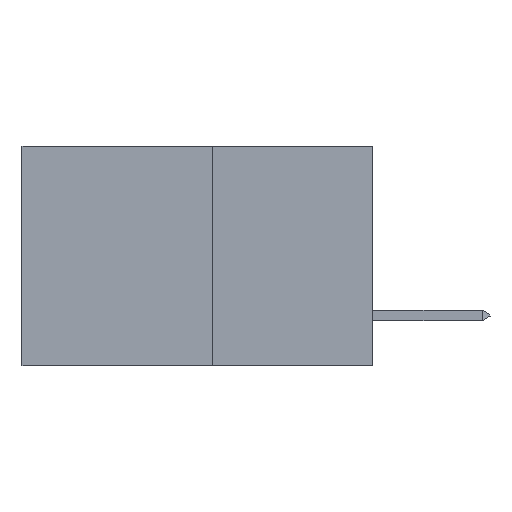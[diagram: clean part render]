
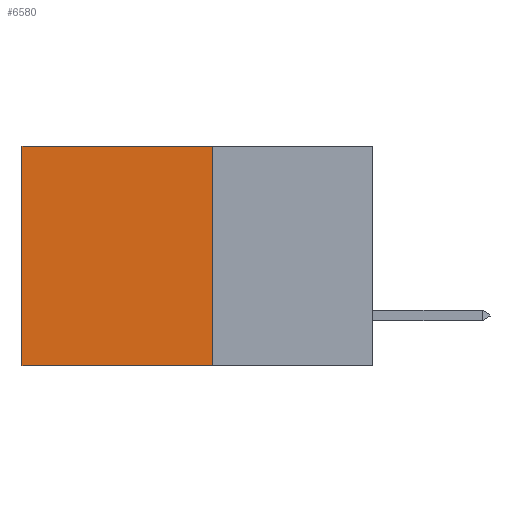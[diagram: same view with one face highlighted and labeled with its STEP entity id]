
A CAD part, left-side view. The second image highlights one B-rep face of the part: STEP entity #6580.
In plain terms, the highlighted planar face has unit normal (-1, 0, 0).
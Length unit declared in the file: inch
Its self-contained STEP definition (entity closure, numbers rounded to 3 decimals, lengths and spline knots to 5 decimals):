
#209 = CARTESIAN_POINT ( 'NONE',  ( 0.277, 0.27, 0. ) ) ;
#249 = VERTEX_POINT ( 'NONE', #7115 ) ;
#510 = CARTESIAN_POINT ( 'NONE',  ( 0.277, 0.59, -0.37 ) ) ;
#636 = DIRECTION ( 'NONE',  ( 0., 0., -1. ) ) ;
#1136 = VECTOR ( 'NONE', #2604, 39.37008 ) ;
#1206 = DIRECTION ( 'NONE',  ( 0., 1., 0. ) ) ;
#1592 = CARTESIAN_POINT ( 'NONE',  ( 0.277, 0.27, -0.37 ) ) ;
#1819 = VERTEX_POINT ( 'NONE', #1592 ) ;
#1961 = LINE ( 'NONE', #8917, #9792 ) ;
#2604 = DIRECTION ( 'NONE',  ( 0., 1., 0. ) ) ;
#2756 = VECTOR ( 'NONE', #636, 39.37008 ) ;
#2848 = CARTESIAN_POINT ( 'NONE',  ( 0.277, 0.27, -0.37 ) ) ;
#3018 = DIRECTION ( 'NONE',  ( 0., 0., -1. ) ) ;
#3955 = CARTESIAN_POINT ( 'NONE',  ( 0.277, 0.27, 0. ) ) ;
#4594 = LINE ( 'NONE', #209, #9768 ) ;
#4894 = FACE_OUTER_BOUND ( 'NONE', #5281, .T. ) ;
#5181 = EDGE_CURVE ( 'NONE', #249, #9066, #10531, .T. ) ;
#5281 = EDGE_LOOP ( 'NONE', ( #8452, #8557, #8600, #8949 ) ) ;
#6580 = ADVANCED_FACE ( 'NONE', ( #4894 ), #8913, .F. ) ;
#7115 = CARTESIAN_POINT ( 'NONE',  ( 0.277, 0.59, 0. ) ) ;
#7126 = EDGE_CURVE ( 'NONE', #1819, #9066, #11793, .T. ) ;
#7785 = VERTEX_POINT ( 'NONE', #3955 ) ;
#8433 = EDGE_CURVE ( 'NONE', #7785, #1819, #1961, .T. ) ;
#8452 = ORIENTED_EDGE ( 'NONE', *, *, #5181, .T. ) ;
#8557 = ORIENTED_EDGE ( 'NONE', *, *, #7126, .F. ) ;
#8600 = ORIENTED_EDGE ( 'NONE', *, *, #8433, .F. ) ;
#8747 = DIRECTION ( 'NONE',  ( 0., 0., -1. ) ) ;
#8776 = DIRECTION ( 'NONE',  ( 1., 0., 0. ) ) ;
#8913 = PLANE ( 'NONE',  #11693 ) ;
#8917 = CARTESIAN_POINT ( 'NONE',  ( 0.277, 0.27, -0.37 ) ) ;
#8949 = ORIENTED_EDGE ( 'NONE', *, *, #12287, .T. ) ;
#9066 = VERTEX_POINT ( 'NONE', #10926 ) ;
#9341 = CARTESIAN_POINT ( 'NONE',  ( 0.277, 0.27, -0.37 ) ) ;
#9768 = VECTOR ( 'NONE', #1206, 39.37008 ) ;
#9792 = VECTOR ( 'NONE', #3018, 39.37008 ) ;
#10531 = LINE ( 'NONE', #510, #2756 ) ;
#10926 = CARTESIAN_POINT ( 'NONE',  ( 0.277, 0.59, -0.37 ) ) ;
#11693 = AXIS2_PLACEMENT_3D ( 'NONE', #9341, #8776, #8747 ) ;
#11793 = LINE ( 'NONE', #2848, #1136 ) ;
#12287 = EDGE_CURVE ( 'NONE', #7785, #249, #4594, .T. ) ;
